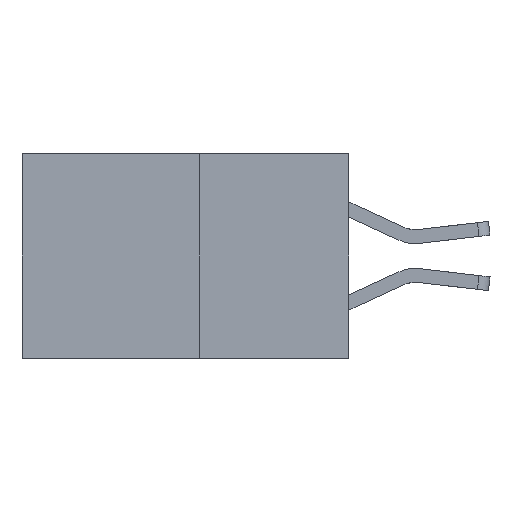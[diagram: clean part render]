
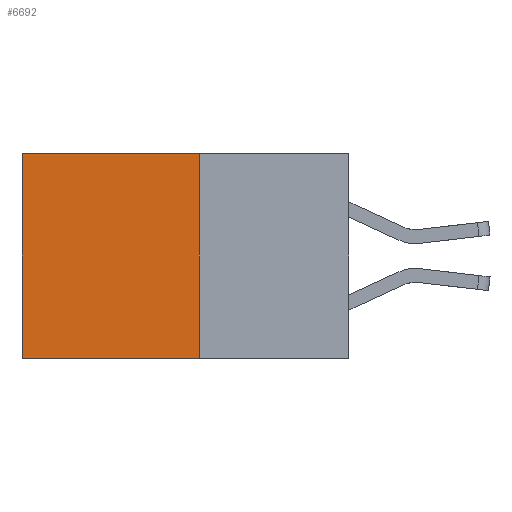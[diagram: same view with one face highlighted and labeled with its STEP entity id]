
A CAD part, left-side view. The second image highlights one B-rep face of the part: STEP entity #6692.
In plain terms, the highlighted planar face has unit normal (-1, 0, 0).
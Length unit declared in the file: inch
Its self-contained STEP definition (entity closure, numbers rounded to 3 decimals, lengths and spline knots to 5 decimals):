
#31 = VECTOR ( 'NONE', #5885, 39.37008 ) ;
#567 = DIRECTION ( 'NONE',  ( 0., 0., -1. ) ) ;
#603 = CARTESIAN_POINT ( 'NONE',  ( 0.277, 0.59, -0.37 ) ) ;
#942 = DIRECTION ( 'NONE',  ( 0., 1., 0. ) ) ;
#1102 = ORIENTED_EDGE ( 'NONE', *, *, #3049, .F. ) ;
#1399 = CARTESIAN_POINT ( 'NONE',  ( 0.277, 0.27, 0. ) ) ;
#1457 = CARTESIAN_POINT ( 'NONE',  ( 0.277, 0.27, -0.37 ) ) ;
#1945 = VECTOR ( 'NONE', #567, 39.37008 ) ;
#1970 = VERTEX_POINT ( 'NONE', #4952 ) ;
#2299 = VECTOR ( 'NONE', #942, 39.37008 ) ;
#2401 = EDGE_LOOP ( 'NONE', ( #10304, #1102, #4803, #6341 ) ) ;
#2584 = VERTEX_POINT ( 'NONE', #1399 ) ;
#2589 = DIRECTION ( 'NONE',  ( 0., 0., -1. ) ) ;
#2608 = CARTESIAN_POINT ( 'NONE',  ( 0.277, 0.27, -0.37 ) ) ;
#2621 = AXIS2_PLACEMENT_3D ( 'NONE', #8056, #7894, #7892 ) ;
#3049 = EDGE_CURVE ( 'NONE', #10609, #1970, #7010, .T. ) ;
#3598 = VECTOR ( 'NONE', #2589, 39.37008 ) ;
#3901 = LINE ( 'NONE', #2608, #3598 ) ;
#4424 = LINE ( 'NONE', #603, #1945 ) ;
#4803 = ORIENTED_EDGE ( 'NONE', *, *, #5629, .F. ) ;
#4952 = CARTESIAN_POINT ( 'NONE',  ( 0.277, 0.59, -0.37 ) ) ;
#5629 = EDGE_CURVE ( 'NONE', #2584, #10609, #3901, .T. ) ;
#5813 = CARTESIAN_POINT ( 'NONE',  ( 0.277, 0.27, -0.37 ) ) ;
#5835 = CARTESIAN_POINT ( 'NONE',  ( 0.277, 0.59, 0. ) ) ;
#5885 = DIRECTION ( 'NONE',  ( 0., 1., 0. ) ) ;
#6341 = ORIENTED_EDGE ( 'NONE', *, *, #10691, .T. ) ;
#6377 = EDGE_CURVE ( 'NONE', #6832, #1970, #4424, .T. ) ;
#6692 = ADVANCED_FACE ( 'NONE', ( #10241 ), #8029, .F. ) ;
#6832 = VERTEX_POINT ( 'NONE', #5835 ) ;
#7010 = LINE ( 'NONE', #1457, #2299 ) ;
#7892 = DIRECTION ( 'NONE',  ( 0., 0., -1. ) ) ;
#7894 = DIRECTION ( 'NONE',  ( 1., 0., 0. ) ) ;
#8029 = PLANE ( 'NONE',  #2621 ) ;
#8056 = CARTESIAN_POINT ( 'NONE',  ( 0.277, 0.27, -0.37 ) ) ;
#9308 = CARTESIAN_POINT ( 'NONE',  ( 0.277, 0.27, 0. ) ) ;
#9550 = LINE ( 'NONE', #9308, #31 ) ;
#10241 = FACE_OUTER_BOUND ( 'NONE', #2401, .T. ) ;
#10304 = ORIENTED_EDGE ( 'NONE', *, *, #6377, .T. ) ;
#10609 = VERTEX_POINT ( 'NONE', #5813 ) ;
#10691 = EDGE_CURVE ( 'NONE', #2584, #6832, #9550, .T. ) ;
